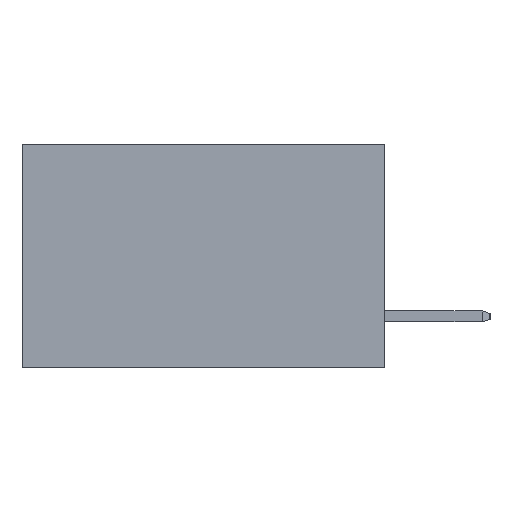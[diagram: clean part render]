
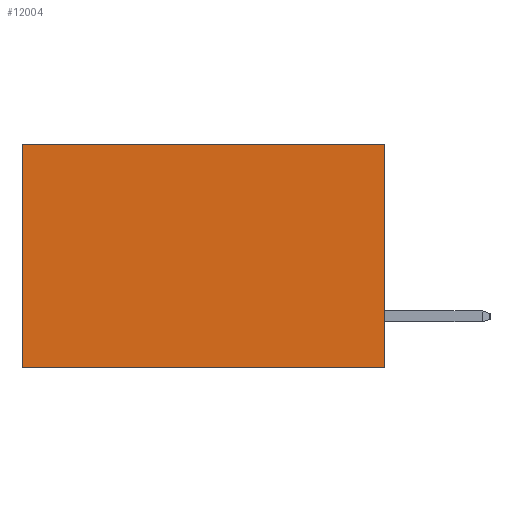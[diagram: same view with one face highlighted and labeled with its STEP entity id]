
A CAD part, left-side view. The second image highlights one B-rep face of the part: STEP entity #12004.
In plain terms, the highlighted planar face has unit normal (-1, 0, 0).
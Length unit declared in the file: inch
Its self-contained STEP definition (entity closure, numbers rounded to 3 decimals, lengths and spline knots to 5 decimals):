
#476 = VERTEX_POINT ( 'NONE', #18746 ) ;
#1709 = VECTOR ( 'NONE', #10250, 39.37008 ) ;
#1777 = LINE ( 'NONE', #4420, #6038 ) ;
#1988 = VERTEX_POINT ( 'NONE', #5067 ) ;
#3308 = CARTESIAN_POINT ( 'NONE',  ( 0.2615, 0., -0.37 ) ) ;
#3706 = CARTESIAN_POINT ( 'NONE',  ( 0.2615, 0., 0. ) ) ;
#4285 = DIRECTION ( 'NONE',  ( 0., 1., 0. ) ) ;
#4420 = CARTESIAN_POINT ( 'NONE',  ( 0.2615, 0., -0.37 ) ) ;
#4605 = FACE_OUTER_BOUND ( 'NONE', #21957, .T. ) ;
#5067 = CARTESIAN_POINT ( 'NONE',  ( 0.2615, 0.6, 0. ) ) ;
#6038 = VECTOR ( 'NONE', #4285, 39.37008 ) ;
#6217 = ORIENTED_EDGE ( 'NONE', *, *, #16118, .T. ) ;
#8845 = DIRECTION ( 'NONE',  ( 0., 0., -1. ) ) ;
#9039 = CARTESIAN_POINT ( 'NONE',  ( 0.2615, 0., -0.37 ) ) ;
#9272 = DIRECTION ( 'NONE',  ( 1., 0., 0. ) ) ;
#9294 = PLANE ( 'NONE',  #18289 ) ;
#9991 = ORIENTED_EDGE ( 'NONE', *, *, #14896, .T. ) ;
#10250 = DIRECTION ( 'NONE',  ( 0., 0., -1. ) ) ;
#10488 = CARTESIAN_POINT ( 'NONE',  ( 0.2615, 0.6, -0.37 ) ) ;
#10976 = LINE ( 'NONE', #3308, #15612 ) ;
#11235 = LINE ( 'NONE', #10488, #1709 ) ;
#12004 = ADVANCED_FACE ( 'NONE', ( #4605 ), #9294, .F. ) ;
#13464 = DIRECTION ( 'NONE',  ( 0., 1., 0. ) ) ;
#13485 = CARTESIAN_POINT ( 'NONE',  ( 0.2615, 0., 0. ) ) ;
#13670 = EDGE_CURVE ( 'NONE', #476, #19689, #1777, .T. ) ;
#14656 = CARTESIAN_POINT ( 'NONE',  ( 0.2615, 0.6, -0.37 ) ) ;
#14896 = EDGE_CURVE ( 'NONE', #1988, #19689, #11235, .T. ) ;
#15612 = VECTOR ( 'NONE', #22431, 39.37008 ) ;
#16118 = EDGE_CURVE ( 'NONE', #18932, #1988, #16905, .T. ) ;
#16376 = VECTOR ( 'NONE', #13464, 39.37008 ) ;
#16812 = ORIENTED_EDGE ( 'NONE', *, *, #20839, .F. ) ;
#16905 = LINE ( 'NONE', #13485, #16376 ) ;
#17452 = ORIENTED_EDGE ( 'NONE', *, *, #13670, .F. ) ;
#18289 = AXIS2_PLACEMENT_3D ( 'NONE', #9039, #9272, #8845 ) ;
#18746 = CARTESIAN_POINT ( 'NONE',  ( 0.2615, 0., -0.37 ) ) ;
#18932 = VERTEX_POINT ( 'NONE', #3706 ) ;
#19689 = VERTEX_POINT ( 'NONE', #14656 ) ;
#20839 = EDGE_CURVE ( 'NONE', #18932, #476, #10976, .T. ) ;
#21957 = EDGE_LOOP ( 'NONE', ( #9991, #17452, #16812, #6217 ) ) ;
#22431 = DIRECTION ( 'NONE',  ( 0., 0., -1. ) ) ;
